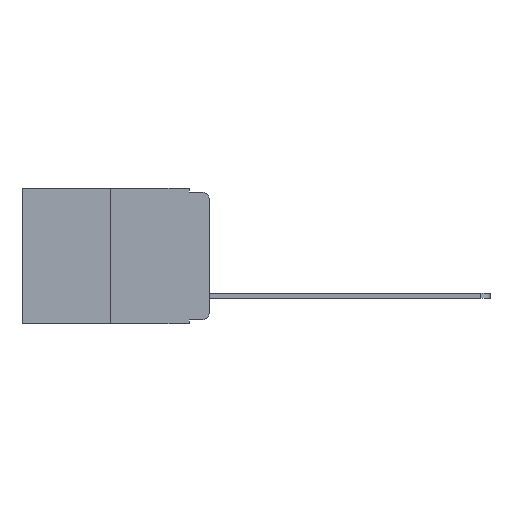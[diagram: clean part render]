
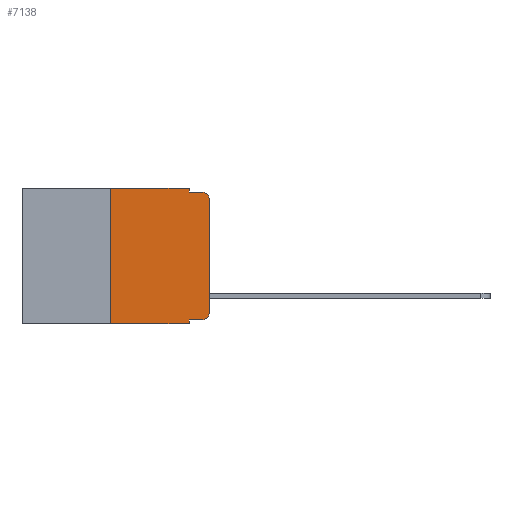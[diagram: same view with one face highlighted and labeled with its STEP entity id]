
A CAD part, left-side view. The second image highlights one B-rep face of the part: STEP entity #7138.
In plain terms, the highlighted planar face has unit normal (-1, 0, 0).
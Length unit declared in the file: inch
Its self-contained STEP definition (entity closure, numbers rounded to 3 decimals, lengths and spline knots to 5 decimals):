
#207 = FACE_OUTER_BOUND ( 'NONE', #1973, .T. ) ;
#361 = DIRECTION ( 'NONE',  ( -1., 0., 0. ) ) ;
#364 = DIRECTION ( 'NONE',  ( 0., 0., -1. ) ) ;
#435 = DIRECTION ( 'NONE',  ( 0., 0., 1. ) ) ;
#458 = CARTESIAN_POINT ( 'NONE',  ( 0., 0., 0. ) ) ;
#522 = CARTESIAN_POINT ( 'NONE',  ( 0., 0.02, -0.03 ) ) ;
#611 = VERTEX_POINT ( 'NONE', #8119 ) ;
#670 = CARTESIAN_POINT ( 'NONE',  ( 0., 0.02, -0.333 ) ) ;
#1334 = EDGE_CURVE ( 'NONE', #3762, #5235, #4831, .T. ) ;
#1645 = EDGE_CURVE ( 'NONE', #5483, #4780, #9530, .T. ) ;
#1739 = VECTOR ( 'NONE', #8813, 39.37008 ) ;
#1791 = VECTOR ( 'NONE', #2391, 39.37008 ) ;
#1855 = EDGE_CURVE ( 'NONE', #3920, #4382, #8655, .T. ) ;
#1858 = EDGE_CURVE ( 'NONE', #4382, #611, #4953, .T. ) ;
#1872 = EDGE_CURVE ( 'NONE', #5235, #4579, #8467, .T. ) ;
#1890 = EDGE_CURVE ( 'NONE', #5483, #3762, #9659, .T. ) ;
#1895 = EDGE_CURVE ( 'NONE', #4307, #2432, #8299, .T. ) ;
#1906 = EDGE_CURVE ( 'NONE', #2432, #3920, #9524, .T. ) ;
#1973 = EDGE_LOOP ( 'NONE', ( #3822, #3831, #3838, #3844, #3850, #3860, #3862, #3873, #3879, #3897 ) ) ;
#2275 = CARTESIAN_POINT ( 'NONE',  ( 0., 0.25, 0. ) ) ;
#2391 = DIRECTION ( 'NONE',  ( 0., -1., 0. ) ) ;
#2432 = VERTEX_POINT ( 'NONE', #670 ) ;
#2548 = CARTESIAN_POINT ( 'NONE',  ( 0., 0.473, -0.343 ) ) ;
#2634 = VECTOR ( 'NONE', #435, 39.37008 ) ;
#2740 = CARTESIAN_POINT ( 'NONE',  ( 0., 0.051, -0.343 ) ) ;
#3017 = AXIS2_PLACEMENT_3D ( 'NONE', #4120, #9043, #4998 ) ;
#3185 = CARTESIAN_POINT ( 'NONE',  ( 0., 0., -0.313 ) ) ;
#3762 = VERTEX_POINT ( 'NONE', #2275 ) ;
#3822 = ORIENTED_EDGE ( 'NONE', *, *, #1855, .T. ) ;
#3831 = ORIENTED_EDGE ( 'NONE', *, *, #1858, .T. ) ;
#3838 = ORIENTED_EDGE ( 'NONE', *, *, #7182, .F. ) ;
#3844 = ORIENTED_EDGE ( 'NONE', *, *, #1872, .F. ) ;
#3850 = ORIENTED_EDGE ( 'NONE', *, *, #1334, .F. ) ;
#3860 = ORIENTED_EDGE ( 'NONE', *, *, #1890, .F. ) ;
#3862 = ORIENTED_EDGE ( 'NONE', *, *, #1645, .T. ) ;
#3873 = ORIENTED_EDGE ( 'NONE', *, *, #6936, .F. ) ;
#3879 = ORIENTED_EDGE ( 'NONE', *, *, #1895, .T. ) ;
#3897 = ORIENTED_EDGE ( 'NONE', *, *, #1906, .T. ) ;
#3920 = VERTEX_POINT ( 'NONE', #3185 ) ;
#4083 = PLANE ( 'NONE',  #3017 ) ;
#4120 = CARTESIAN_POINT ( 'NONE',  ( 0., 0.473, 0. ) ) ;
#4307 = VERTEX_POINT ( 'NONE', #7785 ) ;
#4382 = VERTEX_POINT ( 'NONE', #6657 ) ;
#4406 = VECTOR ( 'NONE', #8938, 39.37008 ) ;
#4579 = VERTEX_POINT ( 'NONE', #6551 ) ;
#4780 = VERTEX_POINT ( 'NONE', #2740 ) ;
#4831 = LINE ( 'NONE', #9200, #9733 ) ;
#4953 = CIRCLE ( 'NONE', #6832, 0.02 ) ;
#4998 = DIRECTION ( 'NONE',  ( 0., 0., -1. ) ) ;
#5235 = VERTEX_POINT ( 'NONE', #7167 ) ;
#5483 = VERTEX_POINT ( 'NONE', #7658 ) ;
#5863 = CARTESIAN_POINT ( 'NONE',  ( 0., 0.051, -0.01 ) ) ;
#6240 = CARTESIAN_POINT ( 'NONE',  ( 0., 0.051, 0. ) ) ;
#6551 = CARTESIAN_POINT ( 'NONE',  ( 0., 0.051, -0.01 ) ) ;
#6657 = CARTESIAN_POINT ( 'NONE',  ( 0., 0., -0.03 ) ) ;
#6832 = AXIS2_PLACEMENT_3D ( 'NONE', #522, #361, #364 ) ;
#6835 = VECTOR ( 'NONE', #8868, 39.37008 ) ;
#6936 = EDGE_CURVE ( 'NONE', #4307, #4780, #8094, .T. ) ;
#7070 = VECTOR ( 'NONE', #9634, 39.37008 ) ;
#7138 = ADVANCED_FACE ( 'NONE', ( #207 ), #4083, .F. ) ;
#7167 = CARTESIAN_POINT ( 'NONE',  ( 0., 0.051, 0. ) ) ;
#7182 = EDGE_CURVE ( 'NONE', #4579, #611, #8435, .T. ) ;
#7441 = CARTESIAN_POINT ( 'NONE',  ( 0., 0.25, 0. ) ) ;
#7658 = CARTESIAN_POINT ( 'NONE',  ( 0., 0.25, -0.343 ) ) ;
#7785 = CARTESIAN_POINT ( 'NONE',  ( 0., 0.051, -0.333 ) ) ;
#8094 = LINE ( 'NONE', #6240, #1739 ) ;
#8119 = CARTESIAN_POINT ( 'NONE',  ( 0., 0.02, -0.01 ) ) ;
#8299 = LINE ( 'NONE', #9229, #4406 ) ;
#8312 = DIRECTION ( 'NONE',  ( 0., 0., -1. ) ) ;
#8435 = LINE ( 'NONE', #5863, #9764 ) ;
#8467 = LINE ( 'NONE', #9496, #7070 ) ;
#8517 = DIRECTION ( 'NONE',  ( 0., -1., 0. ) ) ;
#8655 = LINE ( 'NONE', #458, #2634 ) ;
#8813 = DIRECTION ( 'NONE',  ( 0., 0., -1. ) ) ;
#8840 = AXIS2_PLACEMENT_3D ( 'NONE', #9762, #9756, #8312 ) ;
#8868 = DIRECTION ( 'NONE',  ( 0., 0., 1. ) ) ;
#8938 = DIRECTION ( 'NONE',  ( 0., -1., 0. ) ) ;
#9043 = DIRECTION ( 'NONE',  ( 1., 0., 0. ) ) ;
#9200 = CARTESIAN_POINT ( 'NONE',  ( 0., 0.473, 0. ) ) ;
#9204 = DIRECTION ( 'NONE',  ( 0., -1., 0. ) ) ;
#9229 = CARTESIAN_POINT ( 'NONE',  ( 0., 0.051, -0.333 ) ) ;
#9496 = CARTESIAN_POINT ( 'NONE',  ( 0., 0.051, 0. ) ) ;
#9524 = CIRCLE ( 'NONE', #8840, 0.02 ) ;
#9530 = LINE ( 'NONE', #2548, #1791 ) ;
#9634 = DIRECTION ( 'NONE',  ( 0., 0., -1. ) ) ;
#9659 = LINE ( 'NONE', #7441, #6835 ) ;
#9733 = VECTOR ( 'NONE', #9204, 39.37008 ) ;
#9756 = DIRECTION ( 'NONE',  ( -1., 0., 0. ) ) ;
#9762 = CARTESIAN_POINT ( 'NONE',  ( 0., 0.02, -0.313 ) ) ;
#9764 = VECTOR ( 'NONE', #8517, 39.37008 ) ;
